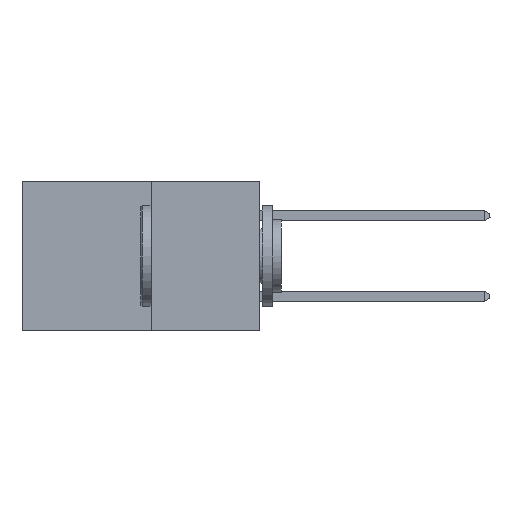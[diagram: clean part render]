
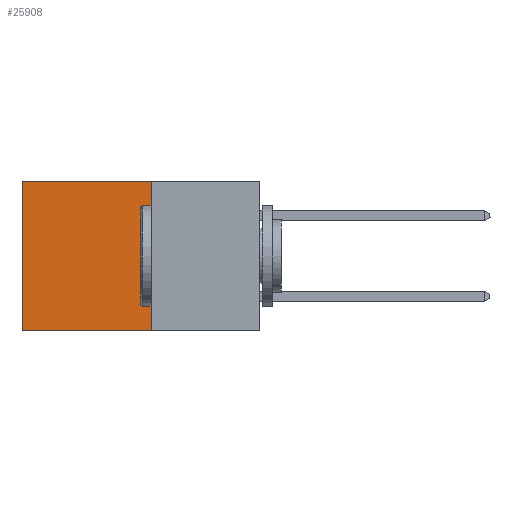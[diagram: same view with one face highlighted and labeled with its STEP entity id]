
A CAD part, left-side view. The second image highlights one B-rep face of the part: STEP entity #25908.
In plain terms, the highlighted planar face has unit normal (-1, 0, 0).
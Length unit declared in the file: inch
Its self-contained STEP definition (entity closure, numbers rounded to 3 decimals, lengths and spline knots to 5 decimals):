
#437 = ORIENTED_EDGE ( 'NONE', *, *, #25955, .T. ) ;
#468 = PLANE ( 'NONE',  #8383 ) ;
#665 = VECTOR ( 'NONE', #2640, 39.37008 ) ;
#1665 = LINE ( 'NONE', #24658, #18296 ) ;
#1873 = CARTESIAN_POINT ( 'NONE',  ( 0.277, 0.27, -0.37 ) ) ;
#2093 = LINE ( 'NONE', #13524, #665 ) ;
#2640 = DIRECTION ( 'NONE',  ( 0., 1., 0. ) ) ;
#3849 = VECTOR ( 'NONE', #26728, 39.37008 ) ;
#4094 = DIRECTION ( 'NONE',  ( 0., 0., -1. ) ) ;
#6888 = EDGE_LOOP ( 'NONE', ( #6920, #13844, #24325, #437 ) ) ;
#6920 = ORIENTED_EDGE ( 'NONE', *, *, #28092, .T. ) ;
#8383 = AXIS2_PLACEMENT_3D ( 'NONE', #20053, #9379, #24385 ) ;
#9379 = DIRECTION ( 'NONE',  ( 1., 0., 0. ) ) ;
#9551 = CARTESIAN_POINT ( 'NONE',  ( 0.277, 0.27, 0. ) ) ;
#9641 = DIRECTION ( 'NONE',  ( 0., 0., -1. ) ) ;
#10270 = VERTEX_POINT ( 'NONE', #15612 ) ;
#11659 = FACE_OUTER_BOUND ( 'NONE', #6888, .T. ) ;
#12706 = VECTOR ( 'NONE', #4094, 39.37008 ) ;
#13524 = CARTESIAN_POINT ( 'NONE',  ( 0.277, 0.27, -0.37 ) ) ;
#13844 = ORIENTED_EDGE ( 'NONE', *, *, #25864, .F. ) ;
#14917 = VERTEX_POINT ( 'NONE', #23175 ) ;
#15612 = CARTESIAN_POINT ( 'NONE',  ( 0.277, 0.27, 0. ) ) ;
#16265 = VERTEX_POINT ( 'NONE', #22405 ) ;
#17860 = VERTEX_POINT ( 'NONE', #23305 ) ;
#18296 = VECTOR ( 'NONE', #9641, 39.37008 ) ;
#19061 = LINE ( 'NONE', #1873, #12706 ) ;
#20053 = CARTESIAN_POINT ( 'NONE',  ( 0.277, 0.27, -0.37 ) ) ;
#21744 = LINE ( 'NONE', #9551, #3849 ) ;
#21849 = EDGE_CURVE ( 'NONE', #10270, #14917, #19061, .T. ) ;
#22405 = CARTESIAN_POINT ( 'NONE',  ( 0.277, 0.59, 0. ) ) ;
#23175 = CARTESIAN_POINT ( 'NONE',  ( 0.277, 0.27, -0.37 ) ) ;
#23305 = CARTESIAN_POINT ( 'NONE',  ( 0.277, 0.59, -0.37 ) ) ;
#24325 = ORIENTED_EDGE ( 'NONE', *, *, #21849, .F. ) ;
#24385 = DIRECTION ( 'NONE',  ( 0., 0., -1. ) ) ;
#24658 = CARTESIAN_POINT ( 'NONE',  ( 0.277, 0.59, -0.37 ) ) ;
#25864 = EDGE_CURVE ( 'NONE', #14917, #17860, #2093, .T. ) ;
#25908 = ADVANCED_FACE ( 'NONE', ( #11659 ), #468, .F. ) ;
#25955 = EDGE_CURVE ( 'NONE', #10270, #16265, #21744, .T. ) ;
#26728 = DIRECTION ( 'NONE',  ( 0., 1., 0. ) ) ;
#28092 = EDGE_CURVE ( 'NONE', #16265, #17860, #1665, .T. ) ;
